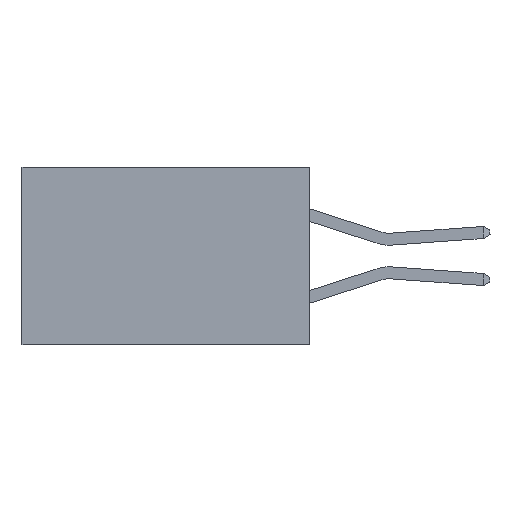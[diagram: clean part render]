
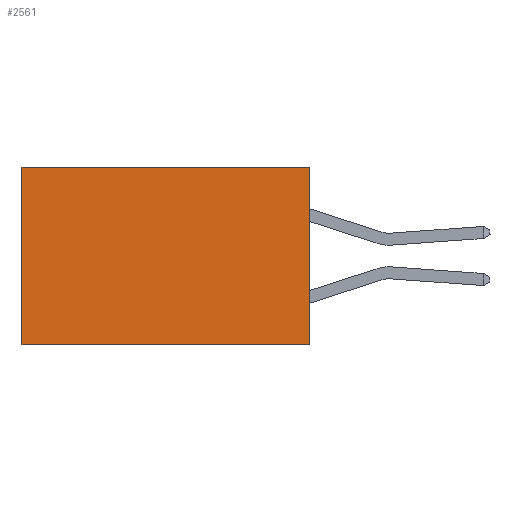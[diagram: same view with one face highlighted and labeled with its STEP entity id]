
A CAD part, left-side view. The second image highlights one B-rep face of the part: STEP entity #2561.
In plain terms, the highlighted planar face has unit normal (-1, 0, 0).
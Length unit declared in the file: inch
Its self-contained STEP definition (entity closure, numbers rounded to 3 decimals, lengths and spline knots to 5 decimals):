
#520 = DIRECTION ( 'NONE',  ( 0., 1., 0. ) ) ;
#548 = VECTOR ( 'NONE', #520, 39.37008 ) ;
#639 = LINE ( 'NONE', #8091, #11555 ) ;
#687 = VERTEX_POINT ( 'NONE', #1745 ) ;
#1568 = CARTESIAN_POINT ( 'NONE',  ( 0.2615, 0., 0. ) ) ;
#1591 = VECTOR ( 'NONE', #6266, 39.37008 ) ;
#1745 = CARTESIAN_POINT ( 'NONE',  ( 0.2615, 0., -0.37 ) ) ;
#2267 = VERTEX_POINT ( 'NONE', #1568 ) ;
#2375 = CARTESIAN_POINT ( 'NONE',  ( 0.2615, 0., -0.37 ) ) ;
#2455 = CARTESIAN_POINT ( 'NONE',  ( 0.2615, 0., -0.37 ) ) ;
#2518 = LINE ( 'NONE', #2455, #548 ) ;
#2561 = ADVANCED_FACE ( 'NONE', ( #9819 ), #7834, .F. ) ;
#2880 = VERTEX_POINT ( 'NONE', #4999 ) ;
#3237 = CARTESIAN_POINT ( 'NONE',  ( 0.2615, 0., -0.37 ) ) ;
#3637 = ORIENTED_EDGE ( 'NONE', *, *, #10266, .F. ) ;
#4976 = DIRECTION ( 'NONE',  ( 1., 0., 0. ) ) ;
#4999 = CARTESIAN_POINT ( 'NONE',  ( 0.2615, 0.6, 0. ) ) ;
#5056 = DIRECTION ( 'NONE',  ( 0., 0., -1. ) ) ;
#5242 = DIRECTION ( 'NONE',  ( 0., 1., 0. ) ) ;
#5564 = VECTOR ( 'NONE', #5056, 39.37008 ) ;
#5797 = VERTEX_POINT ( 'NONE', #6210 ) ;
#6034 = ORIENTED_EDGE ( 'NONE', *, *, #6854, .T. ) ;
#6120 = AXIS2_PLACEMENT_3D ( 'NONE', #3237, #4976, #11628 ) ;
#6210 = CARTESIAN_POINT ( 'NONE',  ( 0.2615, 0.6, -0.37 ) ) ;
#6266 = DIRECTION ( 'NONE',  ( 0., 0., -1. ) ) ;
#6635 = EDGE_CURVE ( 'NONE', #2880, #5797, #11107, .T. ) ;
#6793 = EDGE_CURVE ( 'NONE', #687, #5797, #2518, .T. ) ;
#6854 = EDGE_CURVE ( 'NONE', #2267, #2880, #639, .T. ) ;
#7432 = CARTESIAN_POINT ( 'NONE',  ( 0.2615, 0.6, -0.37 ) ) ;
#7834 = PLANE ( 'NONE',  #6120 ) ;
#8091 = CARTESIAN_POINT ( 'NONE',  ( 0.2615, 0., 0. ) ) ;
#9757 = LINE ( 'NONE', #2375, #1591 ) ;
#9762 = ORIENTED_EDGE ( 'NONE', *, *, #6635, .T. ) ;
#9819 = FACE_OUTER_BOUND ( 'NONE', #9862, .T. ) ;
#9862 = EDGE_LOOP ( 'NONE', ( #9762, #10385, #3637, #6034 ) ) ;
#10266 = EDGE_CURVE ( 'NONE', #2267, #687, #9757, .T. ) ;
#10385 = ORIENTED_EDGE ( 'NONE', *, *, #6793, .F. ) ;
#11107 = LINE ( 'NONE', #7432, #5564 ) ;
#11555 = VECTOR ( 'NONE', #5242, 39.37008 ) ;
#11628 = DIRECTION ( 'NONE',  ( 0., 0., -1. ) ) ;
